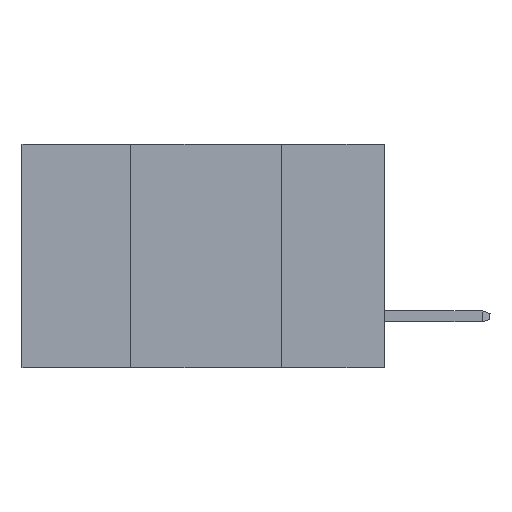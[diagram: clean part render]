
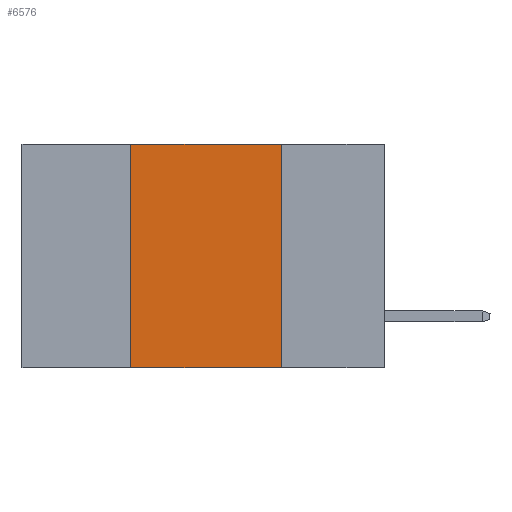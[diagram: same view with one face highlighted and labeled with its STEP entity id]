
A CAD part, left-side view. The second image highlights one B-rep face of the part: STEP entity #6576.
In plain terms, the highlighted planar face has unit normal (-1, 0, 0).
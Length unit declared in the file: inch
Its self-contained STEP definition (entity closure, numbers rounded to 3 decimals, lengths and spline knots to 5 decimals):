
#365 = CARTESIAN_POINT ( 'NONE',  ( 0., 0.6, 0. ) ) ;
#1173 = ORIENTED_EDGE ( 'NONE', *, *, #1290, .F. ) ;
#1231 = EDGE_LOOP ( 'NONE', ( #5822, #1173, #15083, #12463 ) ) ;
#1290 = EDGE_CURVE ( 'NONE', #7295, #3656, #2753, .T. ) ;
#1596 = CARTESIAN_POINT ( 'NONE',  ( 0., 0.42, 0. ) ) ;
#2753 = LINE ( 'NONE', #365, #13836 ) ;
#3331 = DIRECTION ( 'NONE',  ( 0., -1., 0. ) ) ;
#3656 = VERTEX_POINT ( 'NONE', #8236 ) ;
#4921 = VERTEX_POINT ( 'NONE', #10973 ) ;
#5231 = DIRECTION ( 'NONE',  ( 0., -1., 0. ) ) ;
#5555 = PLANE ( 'NONE',  #15562 ) ;
#5698 = LINE ( 'NONE', #10573, #15654 ) ;
#5760 = EDGE_CURVE ( 'NONE', #4921, #6130, #11650, .T. ) ;
#5822 = ORIENTED_EDGE ( 'NONE', *, *, #7075, .F. ) ;
#6130 = VERTEX_POINT ( 'NONE', #6759 ) ;
#6576 = ADVANCED_FACE ( 'NONE', ( #8094 ), #5555, .F. ) ;
#6759 = CARTESIAN_POINT ( 'NONE',  ( 0., 0.17, -0.37 ) ) ;
#7075 = EDGE_CURVE ( 'NONE', #3656, #6130, #5698, .T. ) ;
#7295 = VERTEX_POINT ( 'NONE', #1596 ) ;
#7555 = CARTESIAN_POINT ( 'NONE',  ( 0., 0.42, -0.37 ) ) ;
#8094 = FACE_OUTER_BOUND ( 'NONE', #1231, .T. ) ;
#8236 = CARTESIAN_POINT ( 'NONE',  ( 0., 0.17, 0. ) ) ;
#8283 = CARTESIAN_POINT ( 'NONE',  ( 0., 0.6, -0.37 ) ) ;
#8608 = VECTOR ( 'NONE', #3331, 39.37008 ) ;
#8830 = LINE ( 'NONE', #7555, #15266 ) ;
#10573 = CARTESIAN_POINT ( 'NONE',  ( 0., 0.17, -0.37 ) ) ;
#10591 = DIRECTION ( 'NONE',  ( 0., 0., -1. ) ) ;
#10973 = CARTESIAN_POINT ( 'NONE',  ( 0., 0.42, -0.37 ) ) ;
#11119 = EDGE_CURVE ( 'NONE', #4921, #7295, #8830, .T. ) ;
#11650 = LINE ( 'NONE', #8283, #8608 ) ;
#11770 = CARTESIAN_POINT ( 'NONE',  ( 0., 0.6, 0. ) ) ;
#12414 = DIRECTION ( 'NONE',  ( 0., 0., 1. ) ) ;
#12463 = ORIENTED_EDGE ( 'NONE', *, *, #5760, .T. ) ;
#13836 = VECTOR ( 'NONE', #5231, 39.37008 ) ;
#13894 = DIRECTION ( 'NONE',  ( 0., 0., -1. ) ) ;
#15083 = ORIENTED_EDGE ( 'NONE', *, *, #11119, .F. ) ;
#15109 = DIRECTION ( 'NONE',  ( 1., 0., 0. ) ) ;
#15266 = VECTOR ( 'NONE', #12414, 39.37008 ) ;
#15562 = AXIS2_PLACEMENT_3D ( 'NONE', #11770, #15109, #10591 ) ;
#15654 = VECTOR ( 'NONE', #13894, 39.37008 ) ;
